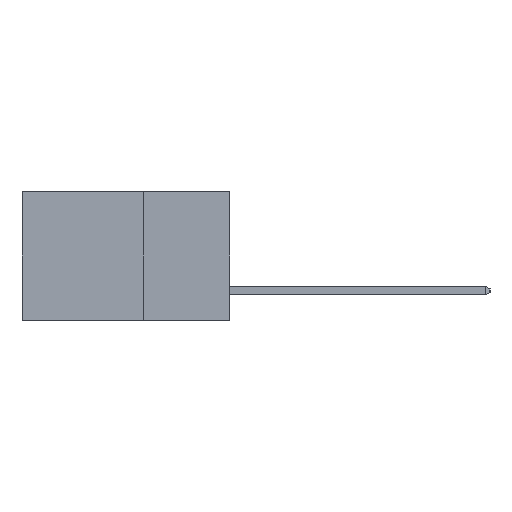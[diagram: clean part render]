
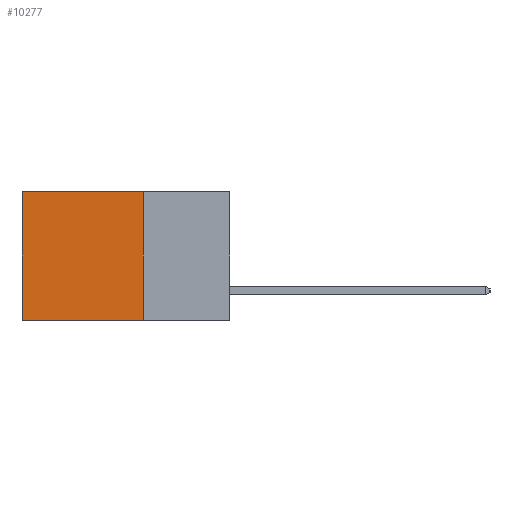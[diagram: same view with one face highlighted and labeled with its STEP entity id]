
A CAD part, left-side view. The second image highlights one B-rep face of the part: STEP entity #10277.
In plain terms, the highlighted planar face has unit normal (-1, 0, 0).
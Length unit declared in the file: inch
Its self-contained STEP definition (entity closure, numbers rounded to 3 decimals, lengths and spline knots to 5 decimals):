
#15 = ORIENTED_EDGE ( 'NONE', *, *, #8114, .F. ) ;
#94 = PLANE ( 'NONE',  #12630 ) ;
#170 = CARTESIAN_POINT ( 'NONE',  ( 0.298, 0.6, 0. ) ) ;
#1172 = VERTEX_POINT ( 'NONE', #11851 ) ;
#1291 = VERTEX_POINT ( 'NONE', #2312 ) ;
#1670 = DIRECTION ( 'NONE',  ( 1., 0., 0. ) ) ;
#2261 = ORIENTED_EDGE ( 'NONE', *, *, #18013, .T. ) ;
#2312 = CARTESIAN_POINT ( 'NONE',  ( 0.298, 0.25, 0. ) ) ;
#4972 = EDGE_CURVE ( 'NONE', #1291, #7118, #11306, .T. ) ;
#5470 = VECTOR ( 'NONE', #18819, 39.37008 ) ;
#5641 = VECTOR ( 'NONE', #16958, 39.37008 ) ;
#5901 = FACE_OUTER_BOUND ( 'NONE', #8219, .T. ) ;
#6154 = LINE ( 'NONE', #18495, #5641 ) ;
#6370 = LINE ( 'NONE', #8916, #18218 ) ;
#7118 = VERTEX_POINT ( 'NONE', #10686 ) ;
#8114 = EDGE_CURVE ( 'NONE', #7118, #1172, #13800, .T. ) ;
#8219 = EDGE_LOOP ( 'NONE', ( #16938, #15, #16873, #2261 ) ) ;
#8916 = CARTESIAN_POINT ( 'NONE',  ( 0.298, 0.25, 0. ) ) ;
#10167 = EDGE_CURVE ( 'NONE', #14377, #1172, #6154, .T. ) ;
#10277 = ADVANCED_FACE ( 'NONE', ( #5901 ), #94, .F. ) ;
#10520 = DIRECTION ( 'NONE',  ( 0., 1., 0. ) ) ;
#10686 = CARTESIAN_POINT ( 'NONE',  ( 0.298, 0.25, -0.37 ) ) ;
#11154 = CARTESIAN_POINT ( 'NONE',  ( 0.298, 0.25, 0. ) ) ;
#11306 = LINE ( 'NONE', #17370, #15826 ) ;
#11812 = CARTESIAN_POINT ( 'NONE',  ( 0.298, 0.25, -0.37 ) ) ;
#11851 = CARTESIAN_POINT ( 'NONE',  ( 0.298, 0.6, -0.37 ) ) ;
#12630 = AXIS2_PLACEMENT_3D ( 'NONE', #11154, #1670, #12715 ) ;
#12715 = DIRECTION ( 'NONE',  ( 0., 0., -1. ) ) ;
#13800 = LINE ( 'NONE', #11812, #5470 ) ;
#14377 = VERTEX_POINT ( 'NONE', #170 ) ;
#15826 = VECTOR ( 'NONE', #17247, 39.37008 ) ;
#16873 = ORIENTED_EDGE ( 'NONE', *, *, #4972, .F. ) ;
#16938 = ORIENTED_EDGE ( 'NONE', *, *, #10167, .T. ) ;
#16958 = DIRECTION ( 'NONE',  ( 0., 0., -1. ) ) ;
#17247 = DIRECTION ( 'NONE',  ( 0., 0., -1. ) ) ;
#17370 = CARTESIAN_POINT ( 'NONE',  ( 0.298, 0.25, 0. ) ) ;
#18013 = EDGE_CURVE ( 'NONE', #1291, #14377, #6370, .T. ) ;
#18218 = VECTOR ( 'NONE', #10520, 39.37008 ) ;
#18495 = CARTESIAN_POINT ( 'NONE',  ( 0.298, 0.6, 0. ) ) ;
#18819 = DIRECTION ( 'NONE',  ( 0., 1., 0. ) ) ;
